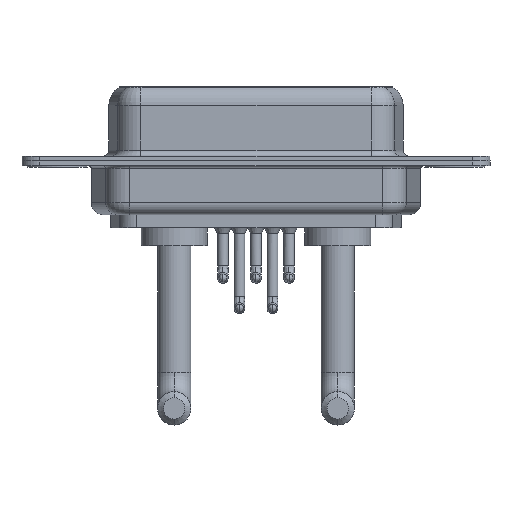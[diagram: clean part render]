
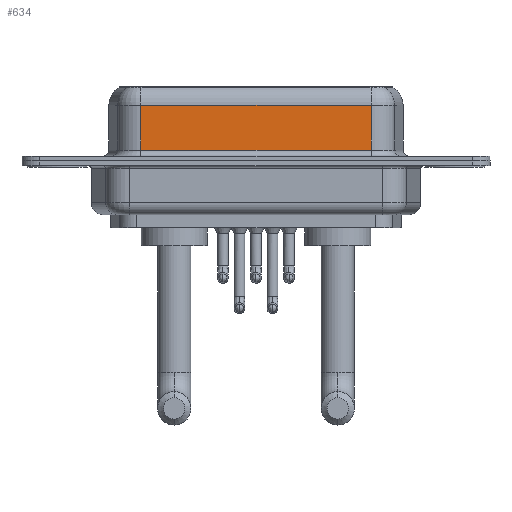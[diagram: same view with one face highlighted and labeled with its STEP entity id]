
A CAD part, front view. The second image highlights one B-rep face of the part: STEP entity #634.
In plain terms, the highlighted planar face has unit normal (0, -1, 0).
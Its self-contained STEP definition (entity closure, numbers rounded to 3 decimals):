
#25 = VECTOR ( 'NONE', #14378, 1000. ) ;
#41 = LINE ( 'NONE', #11524, #10673 ) ;
#97 = VERTEX_POINT ( 'NONE', #3289 ) ;
#101 = CARTESIAN_POINT ( 'NONE',  ( 7.013, -3.95, 4.65 ) ) ;
#502 = DIRECTION ( 'NONE',  ( 0., 0., -1. ) ) ;
#634 = ADVANCED_FACE ( 'NONE', ( #2400 ), #5954, .F. ) ;
#675 = LINE ( 'NONE', #828, #4442 ) ;
#828 = CARTESIAN_POINT ( 'NONE',  ( 26.287, -3.95, 4.65 ) ) ;
#952 = EDGE_CURVE ( 'NONE', #97, #4308, #41, .T. ) ;
#1621 = VERTEX_POINT ( 'NONE', #101 ) ;
#2400 = FACE_OUTER_BOUND ( 'NONE', #6158, .T. ) ;
#3289 = CARTESIAN_POINT ( 'NONE',  ( 7.013, -3.95, 0.9 ) ) ;
#3569 = AXIS2_PLACEMENT_3D ( 'NONE', #10613, #9460, #9241 ) ;
#4308 = VERTEX_POINT ( 'NONE', #14260 ) ;
#4442 = VECTOR ( 'NONE', #10165, 1000. ) ;
#4613 = ORIENTED_EDGE ( 'NONE', *, *, #952, .T. ) ;
#4924 = ORIENTED_EDGE ( 'NONE', *, *, #14484, .T. ) ;
#5954 = PLANE ( 'NONE',  #3569 ) ;
#6158 = EDGE_LOOP ( 'NONE', ( #14224, #4924, #9292, #4613 ) ) ;
#7415 = CARTESIAN_POINT ( 'NONE',  ( 26.287, -3.95, 6.4 ) ) ;
#9241 = DIRECTION ( 'NONE',  ( 0., 0., 1. ) ) ;
#9292 = ORIENTED_EDGE ( 'NONE', *, *, #13820, .T. ) ;
#9303 = DIRECTION ( 'NONE',  ( 1., 0., 0. ) ) ;
#9460 = DIRECTION ( 'NONE',  ( 0., 1., 0. ) ) ;
#10165 = DIRECTION ( 'NONE',  ( -1., 0., 0. ) ) ;
#10516 = CARTESIAN_POINT ( 'NONE',  ( 7.013, -3.95, 6.4 ) ) ;
#10536 = VERTEX_POINT ( 'NONE', #14875 ) ;
#10613 = CARTESIAN_POINT ( 'NONE',  ( 26.287, -3.95, 6.4 ) ) ;
#10673 = VECTOR ( 'NONE', #9303, 1000. ) ;
#11524 = CARTESIAN_POINT ( 'NONE',  ( 26.287, -3.95, 0.9 ) ) ;
#13235 = EDGE_CURVE ( 'NONE', #10536, #4308, #14505, .T. ) ;
#13311 = LINE ( 'NONE', #10516, #25 ) ;
#13820 = EDGE_CURVE ( 'NONE', #1621, #97, #13311, .T. ) ;
#14224 = ORIENTED_EDGE ( 'NONE', *, *, #13235, .F. ) ;
#14260 = CARTESIAN_POINT ( 'NONE',  ( 26.287, -3.95, 0.9 ) ) ;
#14378 = DIRECTION ( 'NONE',  ( 0., 0., -1. ) ) ;
#14484 = EDGE_CURVE ( 'NONE', #10536, #1621, #675, .T. ) ;
#14505 = LINE ( 'NONE', #7415, #14898 ) ;
#14875 = CARTESIAN_POINT ( 'NONE',  ( 26.287, -3.95, 4.65 ) ) ;
#14898 = VECTOR ( 'NONE', #502, 1000. ) ;
